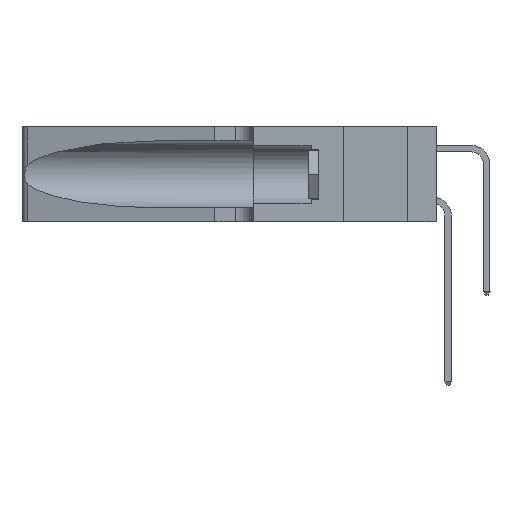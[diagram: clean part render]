
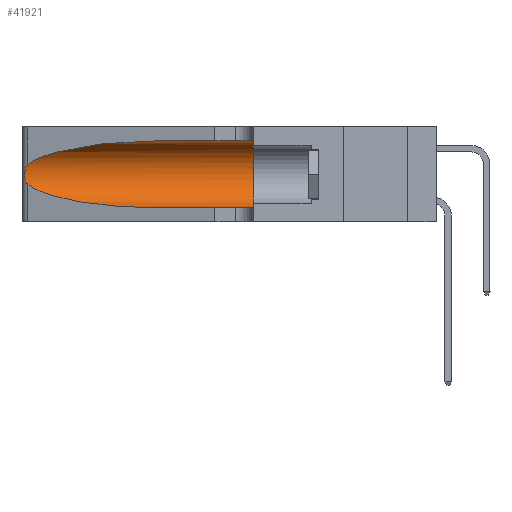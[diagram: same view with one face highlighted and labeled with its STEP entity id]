
A CAD part, left-side view. The second image highlights one B-rep face of the part: STEP entity #41921.
In plain terms, the highlighted cylindrical face has radius 3.308 mm (diameter 6.617 mm), a partial arc.
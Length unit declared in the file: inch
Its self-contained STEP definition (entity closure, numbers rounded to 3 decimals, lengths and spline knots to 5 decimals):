
#1493 = CARTESIAN_POINT ( 'NONE',  ( 0.18966, 0.96281, 0.05475 ) ) ;
#1822 = VERTEX_POINT ( 'NONE', #17990 ) ;
#1954 = CARTESIAN_POINT ( 'NONE',  ( 0.1305, 0.72297, 0.05475 ) ) ;
#2446 = CARTESIAN_POINT ( 'NONE',  ( 0.25787, 1.23484, 0.2124 ) ) ;
#2547 = AXIS2_PLACEMENT_3D ( 'NONE', #44618, #27757, #17467 ) ;
#2588 = CARTESIAN_POINT ( 'NONE',  ( 0.25856, 1.23593, 0.16098 ) ) ;
#3772 = ORIENTED_EDGE ( 'NONE', *, *, #38254, .F. ) ;
#4038 = EDGE_CURVE ( 'NONE', #15736, #6860, #16300, .T. ) ;
#6860 = VERTEX_POINT ( 'NONE', #22061 ) ;
#7297 = CARTESIAN_POINT ( 'NONE',  ( 0.1305, 1.61858, 0.185 ) ) ;
#8357 = CARTESIAN_POINT ( 'NONE',  ( 0.2373, 1.15595, 0.08982 ) ) ;
#8529 = AXIS2_PLACEMENT_3D ( 'NONE', #7297, #37660, #41088 ) ;
#9436 = CARTESIAN_POINT ( 'NONE',  ( 0.25854, 1.2359, 0.20912 ) ) ;
#10770 = VERTEX_POINT ( 'NONE', #18439 ) ;
#11244 = VECTOR ( 'NONE', #25285, 39.37008 ) ;
#13727 = DIRECTION ( 'NONE',  ( 0., -1., 0. ) ) ;
#14739 = ORIENTED_EDGE ( 'NONE', *, *, #26838, .F. ) ;
#15233 = VECTOR ( 'NONE', #13727, 39.37008 ) ;
#15736 = VERTEX_POINT ( 'NONE', #36013 ) ;
#16012 = EDGE_CURVE ( 'NONE', #1822, #37693, #38910, .T. ) ;
#16300 = LINE ( 'NONE', #30815, #15233 ) ;
#16348 = CARTESIAN_POINT ( 'NONE',  ( 0.25555, 1.22993, 0.14849 ) ) ;
#16641 = CARTESIAN_POINT ( 'NONE',  ( 0.26018, 1.23835, 0.19895 ) ) ;
#17374 = CARTESIAN_POINT ( 'NONE',  ( 0.18966, 0.96281, 0.31525 ) ) ;
#17467 = DIRECTION ( 'NONE',  ( 0., 0., 1. ) ) ;
#17990 = CARTESIAN_POINT ( 'NONE',  ( 0.1305, 0.72297, 0.31525 ) ) ;
#18439 = CARTESIAN_POINT ( 'NONE',  ( 0.1305, 0.35, 0.31525 ) ) ;
#19205 = ORIENTED_EDGE ( 'NONE', *, *, #29010, .T. ) ;
#19684 = CARTESIAN_POINT ( 'NONE',  ( 0.25555, 1.22994, 0.2215 ) ) ;
#19825 = CARTESIAN_POINT ( 'NONE',  ( 0.25487, 1.22718, 0.14631 ) ) ;
#20073 = B_SPLINE_CURVE_WITH_KNOTS ( 'NONE', 3,
 ( #36923, #19684, #23169, #2446, #9436, #16641, #30255, #33607, #37218, #2588, #44111, #37073, #16348, #19825 ),
 .UNSPECIFIED., .F., .F.,
 ( 4, 2, 2, 2, 2, 2, 4 ),
 ( 0., 0.00027, 0.00053, 0.00107, 0.0016, 0.00187, 0.00214 ),
 .UNSPECIFIED. ) ;
#20430 = CYLINDRICAL_SURFACE ( 'NONE', #8529, 0.13025 ) ;
#21065 = VERTEX_POINT ( 'NONE', #44220 ) ;
#21106 = ORIENTED_EDGE ( 'NONE', *, *, #16012, .T. ) ;
#21782 = CARTESIAN_POINT ( 'NONE',  ( 0.1305, 1.61858, 0.31525 ) ) ;
#22061 = CARTESIAN_POINT ( 'NONE',  ( 0.1305, 0.35, 0.05475 ) ) ;
#23169 = CARTESIAN_POINT ( 'NONE',  ( 0.25639, 1.23184, 0.21858 ) ) ;
#25285 = DIRECTION ( 'NONE',  ( 0., -1., 0. ) ) ;
#26838 = EDGE_CURVE ( 'NONE', #1822, #10770, #44149, .T. ) ;
#27356 = CARTESIAN_POINT ( 'NONE',  ( 0.25487, 1.22718, 0.22369 ) ) ;
#27499 = CARTESIAN_POINT ( 'NONE',  ( 0.1305, 0.72297, 0.31525 ) ) ;
#27757 = DIRECTION ( 'NONE',  ( 0., 1., 0. ) ) ;
#29010 = EDGE_CURVE ( 'NONE', #21065, #15736, #35601, .T. ) ;
#29024 = CARTESIAN_POINT ( 'NONE',  ( 0.25487, 1.22718, 0.14631 ) ) ;
#30148 = FACE_OUTER_BOUND ( 'NONE', #37386, .T. ) ;
#30255 = CARTESIAN_POINT ( 'NONE',  ( 0.26075, 1.23896, 0.19203 ) ) ;
#30815 = CARTESIAN_POINT ( 'NONE',  ( 0.1305, 1.61858, 0.05475 ) ) ;
#30984 = CARTESIAN_POINT ( 'NONE',  ( 0.25487, 1.22718, 0.22369 ) ) ;
#33607 = CARTESIAN_POINT ( 'NONE',  ( 0.26075, 1.23896, 0.178 ) ) ;
#35271 = ORIENTED_EDGE ( 'NONE', *, *, #4038, .T. ) ;
#35601 =( BOUNDED_CURVE ( )  B_SPLINE_CURVE ( 3, ( #29024, #8357, #1493, #1954 ),
 .UNSPECIFIED., .F., .T. ) 
 B_SPLINE_CURVE_WITH_KNOTS ( ( 4, 4 ),
 ( 3.44316, 4.71239 ),
 .UNSPECIFIED. ) 
 CURVE ( )  GEOMETRIC_REPRESENTATION_ITEM ( )  RATIONAL_B_SPLINE_CURVE ( ( 1., 0.87, 0.87, 1. ) ) 
 REPRESENTATION_ITEM ( '' )  );
#36013 = CARTESIAN_POINT ( 'NONE',  ( 0.1305, 0.72297, 0.05475 ) ) ;
#36923 = CARTESIAN_POINT ( 'NONE',  ( 0.25487, 1.22718, 0.22369 ) ) ;
#37028 = EDGE_CURVE ( 'NONE', #37693, #21065, #20073, .T. ) ;
#37073 = CARTESIAN_POINT ( 'NONE',  ( 0.25639, 1.23186, 0.15144 ) ) ;
#37218 = CARTESIAN_POINT ( 'NONE',  ( 0.26017, 1.23833, 0.17102 ) ) ;
#37386 = EDGE_LOOP ( 'NONE', ( #21106, #44173, #19205, #35271, #3772, #14739 ) ) ;
#37622 = CARTESIAN_POINT ( 'NONE',  ( 0.2373, 1.15595, 0.28018 ) ) ;
#37660 = DIRECTION ( 'NONE',  ( 0., -1., 0. ) ) ;
#37693 = VERTEX_POINT ( 'NONE', #30984 ) ;
#38254 = EDGE_CURVE ( 'NONE', #10770, #6860, #38601, .T. ) ;
#38601 = CIRCLE ( 'NONE', #2547, 0.13025 ) ;
#38910 =( BOUNDED_CURVE ( )  B_SPLINE_CURVE ( 3, ( #27499, #17374, #37622, #27356 ),
 .UNSPECIFIED., .F., .F. ) 
 B_SPLINE_CURVE_WITH_KNOTS ( ( 4, 4 ),
 ( 1.5708, 2.84003 ),
 .UNSPECIFIED. ) 
 CURVE ( )  GEOMETRIC_REPRESENTATION_ITEM ( )  RATIONAL_B_SPLINE_CURVE ( ( 1., 0.87, 0.87, 1. ) ) 
 REPRESENTATION_ITEM ( '' )  );
#41088 = DIRECTION ( 'NONE',  ( 0., 0., -1. ) ) ;
#41921 = ADVANCED_FACE ( 'NONE', ( #30148 ), #20430, .F. ) ;
#44111 = CARTESIAN_POINT ( 'NONE',  ( 0.25789, 1.23486, 0.15765 ) ) ;
#44149 = LINE ( 'NONE', #21782, #11244 ) ;
#44173 = ORIENTED_EDGE ( 'NONE', *, *, #37028, .T. ) ;
#44220 = CARTESIAN_POINT ( 'NONE',  ( 0.25487, 1.22718, 0.14631 ) ) ;
#44618 = CARTESIAN_POINT ( 'NONE',  ( 0.1305, 0.35, 0.185 ) ) ;
